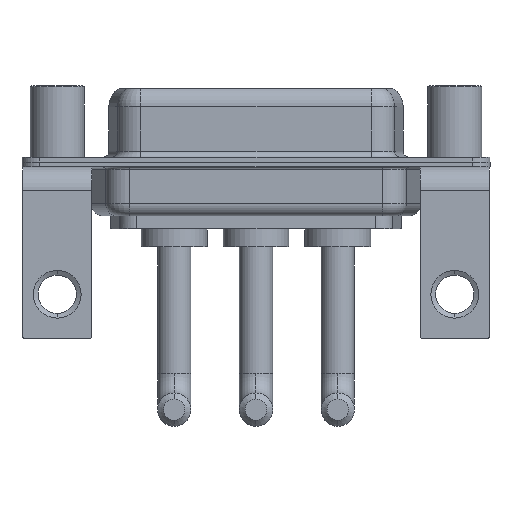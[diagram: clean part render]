
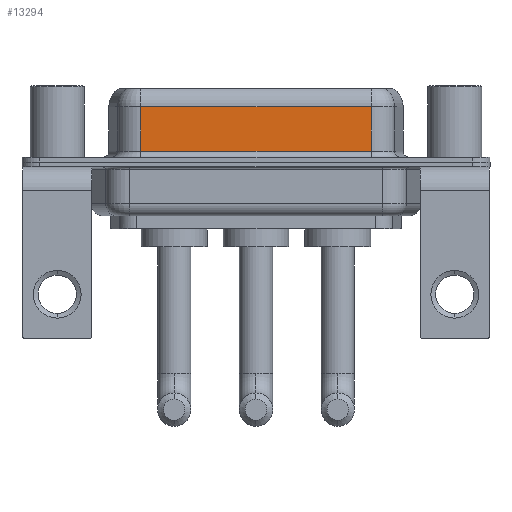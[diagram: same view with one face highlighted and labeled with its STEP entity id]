
A CAD part, front view. The second image highlights one B-rep face of the part: STEP entity #13294.
In plain terms, the highlighted planar face has unit normal (0, -1, 0).
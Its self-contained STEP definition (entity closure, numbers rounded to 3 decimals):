
#99 = VERTEX_POINT ( 'NONE', #11611 ) ;
#223 = ORIENTED_EDGE ( 'NONE', *, *, #11198, .F. ) ;
#434 = ORIENTED_EDGE ( 'NONE', *, *, #7879, .T. ) ;
#465 = LINE ( 'NONE', #11977, #7883 ) ;
#994 = VERTEX_POINT ( 'NONE', #4584 ) ;
#1488 = CARTESIAN_POINT ( 'NONE',  ( 26.287, -3.95, 4.65 ) ) ;
#1522 = CARTESIAN_POINT ( 'NONE',  ( 26.287, -3.95, 6.4 ) ) ;
#1994 = EDGE_LOOP ( 'NONE', ( #223, #434, #6417, #14220 ) ) ;
#2876 = VERTEX_POINT ( 'NONE', #3903 ) ;
#3903 = CARTESIAN_POINT ( 'NONE',  ( 7.013, -3.95, 0.9 ) ) ;
#4420 = DIRECTION ( 'NONE',  ( 0., 0., -1. ) ) ;
#4584 = CARTESIAN_POINT ( 'NONE',  ( 26.287, -3.95, 4.65 ) ) ;
#4770 = CARTESIAN_POINT ( 'NONE',  ( 26.287, -3.95, 0.9 ) ) ;
#5056 = DIRECTION ( 'NONE',  ( 0., 0., -1. ) ) ;
#5087 = VERTEX_POINT ( 'NONE', #13678 ) ;
#5590 = EDGE_CURVE ( 'NONE', #2876, #5087, #13578, .T. ) ;
#6417 = ORIENTED_EDGE ( 'NONE', *, *, #10827, .T. ) ;
#6821 = LINE ( 'NONE', #14799, #8149 ) ;
#7241 = FACE_OUTER_BOUND ( 'NONE', #1994, .T. ) ;
#7321 = DIRECTION ( 'NONE',  ( 0., 0., 1. ) ) ;
#7879 = EDGE_CURVE ( 'NONE', #994, #99, #9681, .T. ) ;
#7883 = VECTOR ( 'NONE', #5056, 1000. ) ;
#8149 = VECTOR ( 'NONE', #4420, 1000. ) ;
#8341 = VECTOR ( 'NONE', #10745, 1000. ) ;
#9681 = LINE ( 'NONE', #1488, #8341 ) ;
#9725 = VECTOR ( 'NONE', #12600, 1000. ) ;
#10699 = DIRECTION ( 'NONE',  ( 0., 1., 0. ) ) ;
#10745 = DIRECTION ( 'NONE',  ( -1., 0., 0. ) ) ;
#10827 = EDGE_CURVE ( 'NONE', #99, #2876, #465, .T. ) ;
#11198 = EDGE_CURVE ( 'NONE', #994, #5087, #6821, .T. ) ;
#11548 = AXIS2_PLACEMENT_3D ( 'NONE', #1522, #10699, #7321 ) ;
#11611 = CARTESIAN_POINT ( 'NONE',  ( 7.013, -3.95, 4.65 ) ) ;
#11830 = PLANE ( 'NONE',  #11548 ) ;
#11977 = CARTESIAN_POINT ( 'NONE',  ( 7.013, -3.95, 6.4 ) ) ;
#12600 = DIRECTION ( 'NONE',  ( 1., 0., 0. ) ) ;
#13294 = ADVANCED_FACE ( 'NONE', ( #7241 ), #11830, .F. ) ;
#13578 = LINE ( 'NONE', #4770, #9725 ) ;
#13678 = CARTESIAN_POINT ( 'NONE',  ( 26.287, -3.95, 0.9 ) ) ;
#14220 = ORIENTED_EDGE ( 'NONE', *, *, #5590, .T. ) ;
#14799 = CARTESIAN_POINT ( 'NONE',  ( 26.287, -3.95, 6.4 ) ) ;
